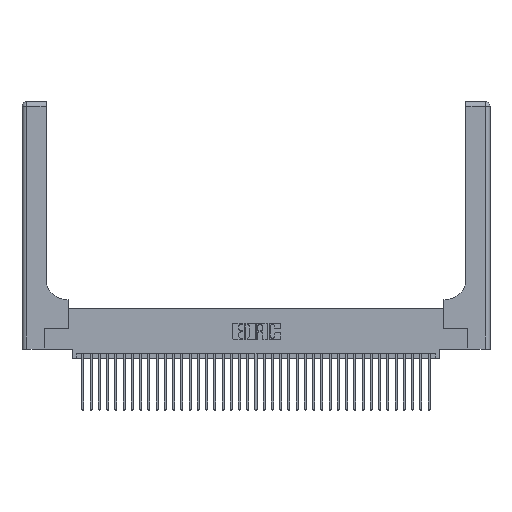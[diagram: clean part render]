
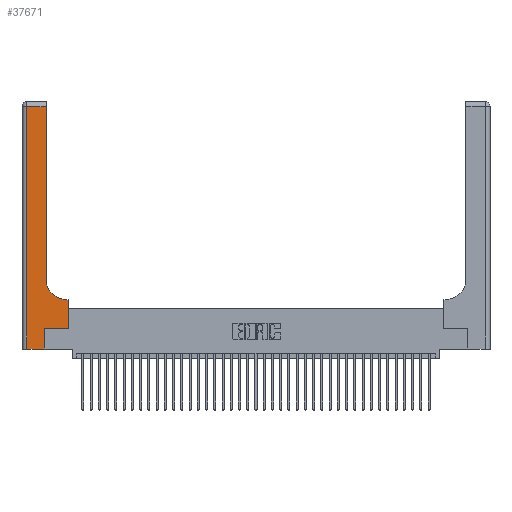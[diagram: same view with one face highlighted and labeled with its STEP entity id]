
A CAD part, top view. The second image highlights one B-rep face of the part: STEP entity #37671.
In plain terms, the highlighted planar face has unit normal (0, 0, 1).
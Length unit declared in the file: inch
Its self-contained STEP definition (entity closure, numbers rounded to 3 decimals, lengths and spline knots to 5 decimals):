
#402 = CARTESIAN_POINT ( 'NONE',  ( 0.5585, 0.25, 0.37 ) ) ;
#2032 = CARTESIAN_POINT ( 'NONE',  ( 0.2915, 2.94, 0.37 ) ) ;
#2063 = CARTESIAN_POINT ( 'NONE',  ( 0., 2.94, 0.37 ) ) ;
#2839 = VECTOR ( 'NONE', #21569, 39.37008 ) ;
#2901 = ORIENTED_EDGE ( 'NONE', *, *, #20914, .T. ) ;
#3606 = ORIENTED_EDGE ( 'NONE', *, *, #32809, .T. ) ;
#4157 = ORIENTED_EDGE ( 'NONE', *, *, #29189, .T. ) ;
#4395 = VECTOR ( 'NONE', #37314, 39.37008 ) ;
#4429 = CARTESIAN_POINT ( 'NONE',  ( 0.06, 3., 0.37 ) ) ;
#4532 = VECTOR ( 'NONE', #12678, 39.37008 ) ;
#5143 = CARTESIAN_POINT ( 'NONE',  ( 0.2915, 3., 0.37 ) ) ;
#5355 = LINE ( 'NONE', #28323, #4395 ) ;
#6586 = VERTEX_POINT ( 'NONE', #7708 ) ;
#6697 = FACE_OUTER_BOUND ( 'NONE', #35777, .T. ) ;
#7708 = CARTESIAN_POINT ( 'NONE',  ( 0.06, 0., 0.37 ) ) ;
#7912 = VERTEX_POINT ( 'NONE', #29578 ) ;
#9266 = AXIS2_PLACEMENT_3D ( 'NONE', #16041, #36921, #19054 ) ;
#9395 = VERTEX_POINT ( 'NONE', #2032 ) ;
#9440 = ORIENTED_EDGE ( 'NONE', *, *, #32887, .T. ) ;
#9737 = ORIENTED_EDGE ( 'NONE', *, *, #19159, .T. ) ;
#9997 = LINE ( 'NONE', #402, #2839 ) ;
#10139 = LINE ( 'NONE', #2063, #33055 ) ;
#11709 = CARTESIAN_POINT ( 'NONE',  ( 0., 3., 0.37 ) ) ;
#12310 = VERTEX_POINT ( 'NONE', #36037 ) ;
#12434 = EDGE_CURVE ( 'NONE', #32642, #29951, #21459, .T. ) ;
#12523 = EDGE_CURVE ( 'NONE', #29951, #27185, #17720, .T. ) ;
#12620 = EDGE_CURVE ( 'NONE', #6586, #7912, #23764, .T. ) ;
#12678 = DIRECTION ( 'NONE',  ( -1., 0., 0. ) ) ;
#13425 = DIRECTION ( 'NONE',  ( 0., -1., 0. ) ) ;
#13689 = DIRECTION ( 'NONE',  ( 1., 0., 0. ) ) ;
#13945 = CARTESIAN_POINT ( 'NONE',  ( 0.2915, 0.85, 0.37 ) ) ;
#14242 = DIRECTION ( 'NONE',  ( 0., 1., 0. ) ) ;
#14416 = ORIENTED_EDGE ( 'NONE', *, *, #14884, .T. ) ;
#14541 = CARTESIAN_POINT ( 'NONE',  ( 0.5415, 0.6, 0.37 ) ) ;
#14884 = EDGE_CURVE ( 'NONE', #27185, #9395, #29646, .T. ) ;
#15932 = CARTESIAN_POINT ( 'NONE',  ( 0.06, 2.94, 0.37 ) ) ;
#16041 = CARTESIAN_POINT ( 'NONE',  ( 0.5415, 0.85, 0.37 ) ) ;
#16056 = CARTESIAN_POINT ( 'NONE',  ( 0.269, 0., 0.37 ) ) ;
#17720 = CIRCLE ( 'NONE', #9266, 0.25 ) ;
#17724 = DIRECTION ( 'NONE',  ( 0., 0., -1. ) ) ;
#19054 = DIRECTION ( 'NONE',  ( 1., 0., 0. ) ) ;
#19159 = EDGE_CURVE ( 'NONE', #9395, #35468, #10139, .T. ) ;
#20190 = DIRECTION ( 'NONE',  ( -1., 0., 0. ) ) ;
#20914 = EDGE_CURVE ( 'NONE', #24170, #32642, #9997, .T. ) ;
#21459 = LINE ( 'NONE', #33422, #4532 ) ;
#21569 = DIRECTION ( 'NONE',  ( 0., 1., 0. ) ) ;
#21722 = VECTOR ( 'NONE', #14242, 39.37008 ) ;
#21897 = VECTOR ( 'NONE', #13689, 39.37008 ) ;
#22253 = ORIENTED_EDGE ( 'NONE', *, *, #12434, .T. ) ;
#23001 = CARTESIAN_POINT ( 'NONE',  ( 0.5585, 0.25, 0.37 ) ) ;
#23764 = LINE ( 'NONE', #28562, #21897 ) ;
#24170 = VERTEX_POINT ( 'NONE', #23001 ) ;
#25713 = ORIENTED_EDGE ( 'NONE', *, *, #12523, .T. ) ;
#27185 = VERTEX_POINT ( 'NONE', #13945 ) ;
#28323 = CARTESIAN_POINT ( 'NONE',  ( 0.269, 0.25, 0.37 ) ) ;
#28562 = CARTESIAN_POINT ( 'NONE',  ( 0., 0., 0.37 ) ) ;
#29189 = EDGE_CURVE ( 'NONE', #35468, #6586, #29489, .T. ) ;
#29489 = LINE ( 'NONE', #4429, #36515 ) ;
#29578 = CARTESIAN_POINT ( 'NONE',  ( 0.269, 0., 0.37 ) ) ;
#29646 = LINE ( 'NONE', #5143, #21722 ) ;
#29951 = VERTEX_POINT ( 'NONE', #14541 ) ;
#31741 = ORIENTED_EDGE ( 'NONE', *, *, #12620, .T. ) ;
#32074 = VECTOR ( 'NONE', #36937, 39.37008 ) ;
#32642 = VERTEX_POINT ( 'NONE', #33175 ) ;
#32809 = EDGE_CURVE ( 'NONE', #7912, #12310, #245, .T. ) ;
#32887 = EDGE_CURVE ( 'NONE', #12310, #24170, #5355, .T. ) ;
#33055 = VECTOR ( 'NONE', #20190, 39.37008 ) ;
#33175 = CARTESIAN_POINT ( 'NONE',  ( 0.5585, 0.6, 0.37 ) ) ;
#33422 = CARTESIAN_POINT ( 'NONE',  ( 0.2915, 0.6, 0.37 ) ) ;
#35072 = AXIS2_PLACEMENT_3D ( 'NONE', #11709, #17724, #38581 ) ;
#35468 = VERTEX_POINT ( 'NONE', #15932 ) ;
#35590 = PLANE ( 'NONE',  #35072 ) ;
#35777 = EDGE_LOOP ( 'NONE', ( #14416, #9737, #4157, #31741, #3606, #9440, #2901, #22253, #25713 ) ) ;
#36037 = CARTESIAN_POINT ( 'NONE',  ( 0.269, 0.25, 0.37 ) ) ;
#36515 = VECTOR ( 'NONE', #13425, 39.37008 ) ;
#36921 = DIRECTION ( 'NONE',  ( 0., 0., -1. ) ) ;
#36937 = DIRECTION ( 'NONE',  ( 0., 1., 0. ) ) ;
#37314 = DIRECTION ( 'NONE',  ( 1., 0., 0. ) ) ;
#37671 = ADVANCED_FACE ( 'NONE', ( #6697 ), #35590, .F. ) ;
#38581 = DIRECTION ( 'NONE',  ( -1., 0., 0. ) ) ;
#245 = LINE ( 'NONE', #16056, #32074 ) ;
